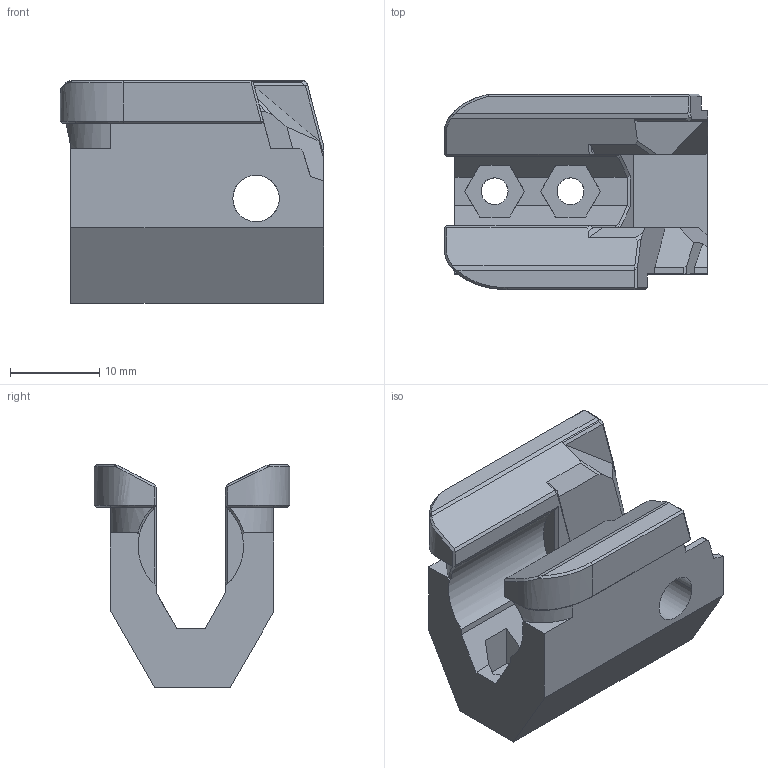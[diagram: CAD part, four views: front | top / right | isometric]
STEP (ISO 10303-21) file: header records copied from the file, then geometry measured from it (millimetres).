
FILE_DESCRIPTION (( 'STEP AP214' ), '1' );
FILE_NAME ('3089 Front Rail Block.STEP', '2022-08-18T00:59:10', ( '' ), ( '' ), 'SwSTEP 2.0', 'SolidWorks 2020', '' );
FILE_SCHEMA (( 'AUTOMOTIVE_DESIGN' ));
Length unit declared in the file: millimetre
Products named in the file (1): 3089 Front Rail Block
Bounding box: 29.44 x 21.89 x 24.95 mm (x, y, z)
Volume: 6454.7 mm3; surface area: 3959.5 mm2
Topology: 1 solids, 1 shells, 134 faces, 390 edges, 256 vertices
Faces by surface type: plane 105, bspline 15, cylinder 12, cone 2
Entity records: 5222 total; most frequent: CARTESIAN_POINT 2071, ORIENTED_EDGE 780, DIRECTION 446, EDGE_CURVE 390, VERTEX_POINT 256, B_SPLINE_CURVE_WITH_KNOTS 197, LINE 170, VECTOR 170
